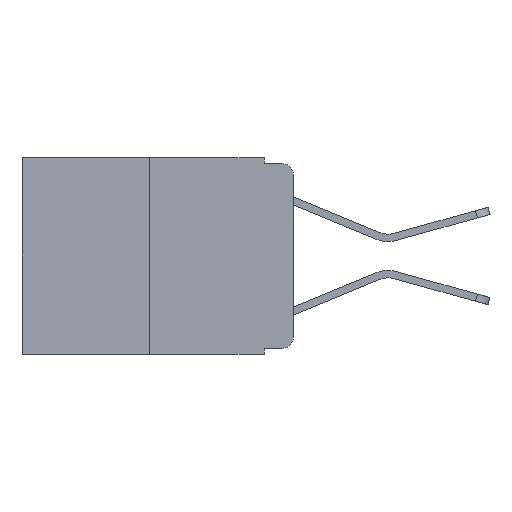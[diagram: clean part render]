
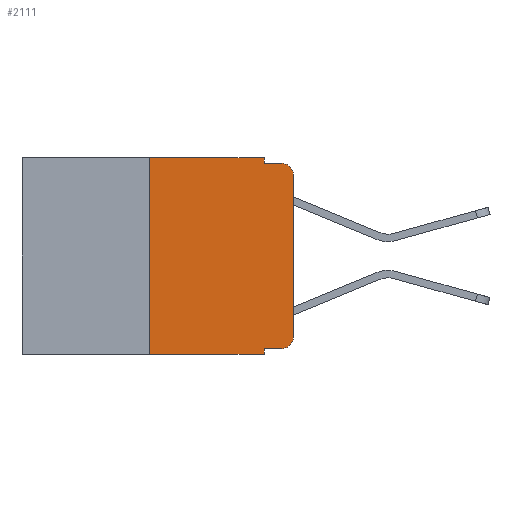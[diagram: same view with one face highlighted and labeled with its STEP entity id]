
A CAD part, left-side view. The second image highlights one B-rep face of the part: STEP entity #2111.
In plain terms, the highlighted planar face has unit normal (-1, 0, 0).
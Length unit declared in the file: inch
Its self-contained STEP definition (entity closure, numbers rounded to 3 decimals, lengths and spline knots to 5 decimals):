
#81 = CARTESIAN_POINT ( 'NONE',  ( 0., 0.051, 0. ) ) ;
#149 = ORIENTED_EDGE ( 'NONE', *, *, #10512, .T. ) ;
#214 = ORIENTED_EDGE ( 'NONE', *, *, #9674, .T. ) ;
#286 = ORIENTED_EDGE ( 'NONE', *, *, #4860, .F. ) ;
#364 = ORIENTED_EDGE ( 'NONE', *, *, #10592, .F. ) ;
#483 = VERTEX_POINT ( 'NONE', #2621 ) ;
#519 = LINE ( 'NONE', #5113, #3218 ) ;
#708 = VECTOR ( 'NONE', #5687, 39.37008 ) ;
#923 = VERTEX_POINT ( 'NONE', #12148 ) ;
#935 = EDGE_CURVE ( 'NONE', #7303, #11316, #6444, .T. ) ;
#939 = VECTOR ( 'NONE', #5622, 39.37008 ) ;
#1136 = ORIENTED_EDGE ( 'NONE', *, *, #4350, .F. ) ;
#1145 = ORIENTED_EDGE ( 'NONE', *, *, #6295, .F. ) ;
#1184 = CARTESIAN_POINT ( 'NONE',  ( 0., 0., -0.03 ) ) ;
#1245 = CIRCLE ( 'NONE', #7849, 0.02 ) ;
#1298 = VERTEX_POINT ( 'NONE', #11696 ) ;
#1551 = ORIENTED_EDGE ( 'NONE', *, *, #935, .F. ) ;
#1674 = CARTESIAN_POINT ( 'NONE',  ( 0., 0.051, -0.333 ) ) ;
#1679 = PLANE ( 'NONE',  #10937 ) ;
#1708 = VECTOR ( 'NONE', #11376, 39.37008 ) ;
#1757 = CARTESIAN_POINT ( 'NONE',  ( 0., 0.473, -0.343 ) ) ;
#2029 = LINE ( 'NONE', #8860, #1708 ) ;
#2111 = ADVANCED_FACE ( 'NONE', ( #6251 ), #1679, .F. ) ;
#2281 = VERTEX_POINT ( 'NONE', #7876 ) ;
#2621 = CARTESIAN_POINT ( 'NONE',  ( 0., 0.02, -0.333 ) ) ;
#2661 = ORIENTED_EDGE ( 'NONE', *, *, #7000, .T. ) ;
#2678 = DIRECTION ( 'NONE',  ( 0., 0., 1. ) ) ;
#2939 = LINE ( 'NONE', #11366, #10123 ) ;
#3218 = VECTOR ( 'NONE', #6143, 39.37008 ) ;
#3329 = ORIENTED_EDGE ( 'NONE', *, *, #4151, .T. ) ;
#3401 = LINE ( 'NONE', #4688, #708 ) ;
#3859 = CARTESIAN_POINT ( 'NONE',  ( 0., 0.473, 0. ) ) ;
#3862 = VECTOR ( 'NONE', #5846, 39.37008 ) ;
#4080 = CARTESIAN_POINT ( 'NONE',  ( 0., 0.051, 0. ) ) ;
#4151 = EDGE_CURVE ( 'NONE', #1298, #4239, #6745, .T. ) ;
#4180 = VECTOR ( 'NONE', #2678, 39.37008 ) ;
#4239 = VERTEX_POINT ( 'NONE', #1184 ) ;
#4350 = EDGE_CURVE ( 'NONE', #2281, #4845, #2029, .T. ) ;
#4688 = CARTESIAN_POINT ( 'NONE',  ( 0., 0.051, -0.01 ) ) ;
#4845 = VERTEX_POINT ( 'NONE', #4080 ) ;
#4860 = EDGE_CURVE ( 'NONE', #6837, #6452, #3401, .T. ) ;
#5039 = DIRECTION ( 'NONE',  ( -1., 0., 0. ) ) ;
#5113 = CARTESIAN_POINT ( 'NONE',  ( 0., 0.051, -0.333 ) ) ;
#5484 = DIRECTION ( 'NONE',  ( -1., 0., 0. ) ) ;
#5542 = AXIS2_PLACEMENT_3D ( 'NONE', #10976, #5484, #11847 ) ;
#5622 = DIRECTION ( 'NONE',  ( 0., -1., 0. ) ) ;
#5687 = DIRECTION ( 'NONE',  ( 0., -1., 0. ) ) ;
#5846 = DIRECTION ( 'NONE',  ( 0., 0., -1. ) ) ;
#6143 = DIRECTION ( 'NONE',  ( 0., -1., 0. ) ) ;
#6186 = LINE ( 'NONE', #1757, #939 ) ;
#6219 = CARTESIAN_POINT ( 'NONE',  ( 0., 0.051, -0.343 ) ) ;
#6251 = FACE_OUTER_BOUND ( 'NONE', #8671, .T. ) ;
#6295 = EDGE_CURVE ( 'NONE', #923, #2281, #2939, .T. ) ;
#6444 = LINE ( 'NONE', #81, #3862 ) ;
#6452 = VERTEX_POINT ( 'NONE', #10702 ) ;
#6686 = ORIENTED_EDGE ( 'NONE', *, *, #10191, .T. ) ;
#6745 = LINE ( 'NONE', #9193, #4180 ) ;
#6837 = VERTEX_POINT ( 'NONE', #7779 ) ;
#7000 = EDGE_CURVE ( 'NONE', #7303, #483, #519, .T. ) ;
#7303 = VERTEX_POINT ( 'NONE', #1674 ) ;
#7767 = LINE ( 'NONE', #10693, #12204 ) ;
#7777 = CIRCLE ( 'NONE', #5542, 0.02 ) ;
#7779 = CARTESIAN_POINT ( 'NONE',  ( 0., 0.051, -0.01 ) ) ;
#7849 = AXIS2_PLACEMENT_3D ( 'NONE', #10579, #5039, #11453 ) ;
#7876 = CARTESIAN_POINT ( 'NONE',  ( 0., 0.25, 0. ) ) ;
#7924 = DIRECTION ( 'NONE',  ( 0., 0., -1. ) ) ;
#7966 = DIRECTION ( 'NONE',  ( 1., 0., 0. ) ) ;
#8671 = EDGE_LOOP ( 'NONE', ( #3329, #149, #286, #364, #1136, #1145, #214, #1551, #2661, #6686 ) ) ;
#8720 = DIRECTION ( 'NONE',  ( 0., 0., 1. ) ) ;
#8860 = CARTESIAN_POINT ( 'NONE',  ( 0., 0.473, 0. ) ) ;
#9193 = CARTESIAN_POINT ( 'NONE',  ( 0., 0., 0. ) ) ;
#9674 = EDGE_CURVE ( 'NONE', #923, #11316, #6186, .T. ) ;
#10123 = VECTOR ( 'NONE', #8720, 39.37008 ) ;
#10191 = EDGE_CURVE ( 'NONE', #483, #1298, #7777, .T. ) ;
#10512 = EDGE_CURVE ( 'NONE', #4239, #6452, #1245, .T. ) ;
#10579 = CARTESIAN_POINT ( 'NONE',  ( 0., 0.02, -0.03 ) ) ;
#10592 = EDGE_CURVE ( 'NONE', #4845, #6837, #7767, .T. ) ;
#10693 = CARTESIAN_POINT ( 'NONE',  ( 0., 0.051, 0. ) ) ;
#10702 = CARTESIAN_POINT ( 'NONE',  ( 0., 0.02, -0.01 ) ) ;
#10937 = AXIS2_PLACEMENT_3D ( 'NONE', #3859, #7966, #7924 ) ;
#10976 = CARTESIAN_POINT ( 'NONE',  ( 0., 0.02, -0.313 ) ) ;
#11316 = VERTEX_POINT ( 'NONE', #6219 ) ;
#11366 = CARTESIAN_POINT ( 'NONE',  ( 0., 0.25, 0. ) ) ;
#11376 = DIRECTION ( 'NONE',  ( 0., -1., 0. ) ) ;
#11453 = DIRECTION ( 'NONE',  ( 0., 0., -1. ) ) ;
#11574 = DIRECTION ( 'NONE',  ( 0., 0., -1. ) ) ;
#11696 = CARTESIAN_POINT ( 'NONE',  ( 0., 0., -0.313 ) ) ;
#11847 = DIRECTION ( 'NONE',  ( 0., 0., -1. ) ) ;
#12148 = CARTESIAN_POINT ( 'NONE',  ( 0., 0.25, -0.343 ) ) ;
#12204 = VECTOR ( 'NONE', #11574, 39.37008 ) ;
